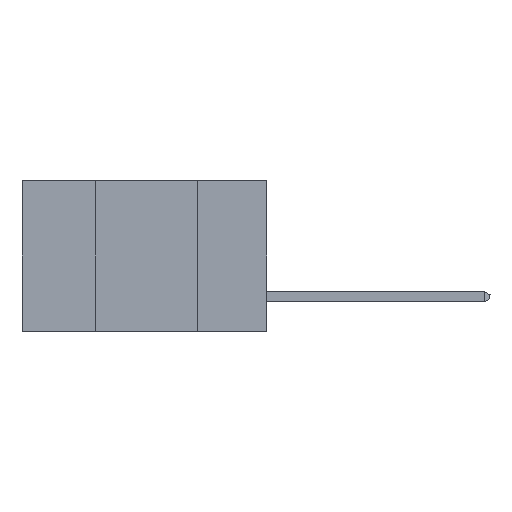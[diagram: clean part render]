
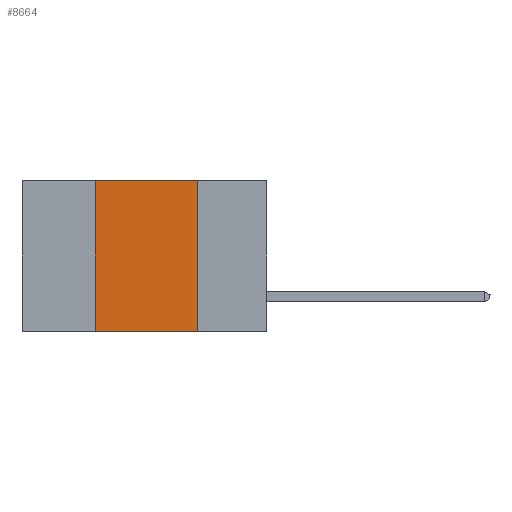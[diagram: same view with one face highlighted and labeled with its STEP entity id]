
A CAD part, left-side view. The second image highlights one B-rep face of the part: STEP entity #8664.
In plain terms, the highlighted planar face has unit normal (-1, 0, 0).
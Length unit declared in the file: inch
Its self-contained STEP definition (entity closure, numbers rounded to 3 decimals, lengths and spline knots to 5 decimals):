
#1714 = VERTEX_POINT ( 'NONE', #16390 ) ;
#1785 = VECTOR ( 'NONE', #18649, 39.37008 ) ;
#2245 = LINE ( 'NONE', #6796, #1785 ) ;
#2336 = EDGE_CURVE ( 'NONE', #7868, #12394, #6353, .T. ) ;
#2399 = DIRECTION ( 'NONE',  ( 1., 0., 0. ) ) ;
#3855 = DIRECTION ( 'NONE',  ( 0., 0., -1. ) ) ;
#4291 = VECTOR ( 'NONE', #17530, 39.37008 ) ;
#4548 = DIRECTION ( 'NONE',  ( 0., -1., 0. ) ) ;
#4565 = AXIS2_PLACEMENT_3D ( 'NONE', #12607, #2399, #3855 ) ;
#4802 = CARTESIAN_POINT ( 'NONE',  ( 0., 0.42, 0. ) ) ;
#5041 = VECTOR ( 'NONE', #4548, 39.37008 ) ;
#5114 = PLANE ( 'NONE',  #4565 ) ;
#5519 = EDGE_CURVE ( 'NONE', #12394, #1714, #11929, .T. ) ;
#6353 = LINE ( 'NONE', #4802, #13813 ) ;
#6441 = ORIENTED_EDGE ( 'NONE', *, *, #5519, .F. ) ;
#6796 = CARTESIAN_POINT ( 'NONE',  ( 0., 0.6, -0.37 ) ) ;
#7868 = VERTEX_POINT ( 'NONE', #13144 ) ;
#8136 = FACE_OUTER_BOUND ( 'NONE', #18056, .T. ) ;
#8664 = ADVANCED_FACE ( 'NONE', ( #8136 ), #5114, .F. ) ;
#8760 = CARTESIAN_POINT ( 'NONE',  ( 0., 0.17, -0.37 ) ) ;
#11121 = EDGE_CURVE ( 'NONE', #1714, #17767, #11512, .T. ) ;
#11379 = ORIENTED_EDGE ( 'NONE', *, *, #2336, .F. ) ;
#11512 = LINE ( 'NONE', #18991, #4291 ) ;
#11928 = ORIENTED_EDGE ( 'NONE', *, *, #13257, .T. ) ;
#11929 = LINE ( 'NONE', #17861, #5041 ) ;
#12394 = VERTEX_POINT ( 'NONE', #16176 ) ;
#12607 = CARTESIAN_POINT ( 'NONE',  ( 0., 0.6, 0. ) ) ;
#13144 = CARTESIAN_POINT ( 'NONE',  ( 0., 0.42, -0.37 ) ) ;
#13257 = EDGE_CURVE ( 'NONE', #7868, #17767, #2245, .T. ) ;
#13368 = ORIENTED_EDGE ( 'NONE', *, *, #11121, .F. ) ;
#13813 = VECTOR ( 'NONE', #16945, 39.37008 ) ;
#16176 = CARTESIAN_POINT ( 'NONE',  ( 0., 0.42, 0. ) ) ;
#16390 = CARTESIAN_POINT ( 'NONE',  ( 0., 0.17, 0. ) ) ;
#16945 = DIRECTION ( 'NONE',  ( 0., 0., 1. ) ) ;
#17530 = DIRECTION ( 'NONE',  ( 0., 0., -1. ) ) ;
#17767 = VERTEX_POINT ( 'NONE', #8760 ) ;
#17861 = CARTESIAN_POINT ( 'NONE',  ( 0., 0.6, 0. ) ) ;
#18056 = EDGE_LOOP ( 'NONE', ( #13368, #6441, #11379, #11928 ) ) ;
#18649 = DIRECTION ( 'NONE',  ( 0., -1., 0. ) ) ;
#18991 = CARTESIAN_POINT ( 'NONE',  ( 0., 0.17, 0. ) ) ;
